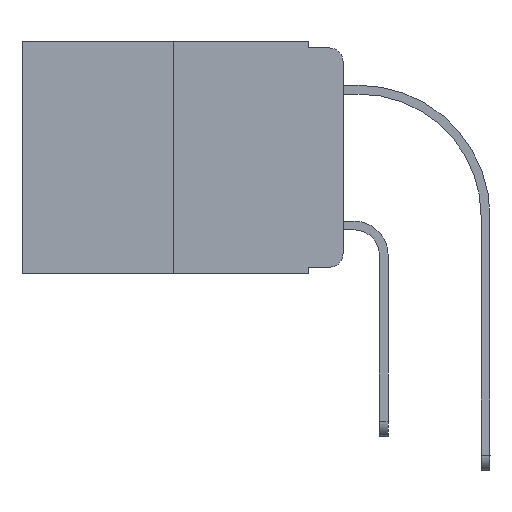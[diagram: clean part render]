
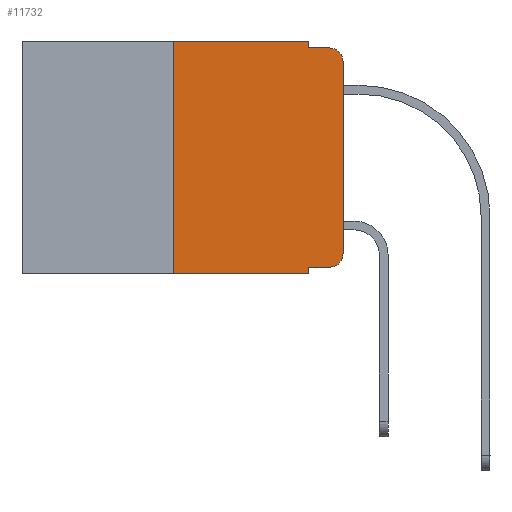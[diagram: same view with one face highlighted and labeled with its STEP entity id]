
A CAD part, left-side view. The second image highlights one B-rep face of the part: STEP entity #11732.
In plain terms, the highlighted planar face has unit normal (-1, 0, 0).
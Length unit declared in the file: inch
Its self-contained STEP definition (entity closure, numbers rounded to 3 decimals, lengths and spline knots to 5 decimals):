
#856 = ORIENTED_EDGE ( 'NONE', *, *, #9718, .F. ) ;
#1304 = EDGE_CURVE ( 'NONE', #6301, #11954, #2735, .T. ) ;
#1431 = EDGE_CURVE ( 'NONE', #22764, #14516, #23906, .T. ) ;
#1926 = DIRECTION ( 'NONE',  ( 0., 0., 1. ) ) ;
#2358 = AXIS2_PLACEMENT_3D ( 'NONE', #17321, #22872, #11988 ) ;
#2363 = DIRECTION ( 'NONE',  ( 0., 0., -1. ) ) ;
#2381 = CARTESIAN_POINT ( 'NONE',  ( 0., 0.02, -0.01 ) ) ;
#2456 = DIRECTION ( 'NONE',  ( -1., 0., 0. ) ) ;
#2527 = AXIS2_PLACEMENT_3D ( 'NONE', #20752, #18953, #2363 ) ;
#2655 = ORIENTED_EDGE ( 'NONE', *, *, #7202, .T. ) ;
#2735 = LINE ( 'NONE', #8079, #3494 ) ;
#2986 = LINE ( 'NONE', #15823, #6838 ) ;
#3075 = LINE ( 'NONE', #19781, #23325 ) ;
#3313 = DIRECTION ( 'NONE',  ( 0., -1., 0. ) ) ;
#3494 = VECTOR ( 'NONE', #6258, 39.37008 ) ;
#3755 = CARTESIAN_POINT ( 'NONE',  ( 0., 0.051, -0.333 ) ) ;
#4298 = FACE_OUTER_BOUND ( 'NONE', #11430, .T. ) ;
#4517 = EDGE_CURVE ( 'NONE', #23279, #20441, #9704, .T. ) ;
#4777 = DIRECTION ( 'NONE',  ( 0., 0., -1. ) ) ;
#4959 = CARTESIAN_POINT ( 'NONE',  ( 0., 0., -0.03 ) ) ;
#5026 = CARTESIAN_POINT ( 'NONE',  ( 0., 0.25, 0. ) ) ;
#5058 = DIRECTION ( 'NONE',  ( 0., 0., 1. ) ) ;
#5303 = VERTEX_POINT ( 'NONE', #19049 ) ;
#5310 = VECTOR ( 'NONE', #1926, 39.37008 ) ;
#6258 = DIRECTION ( 'NONE',  ( 0., -1., 0. ) ) ;
#6301 = VERTEX_POINT ( 'NONE', #22852 ) ;
#6594 = DIRECTION ( 'NONE',  ( 0., -1., 0. ) ) ;
#6620 = VERTEX_POINT ( 'NONE', #2381 ) ;
#6838 = VECTOR ( 'NONE', #5058, 39.37008 ) ;
#7202 = EDGE_CURVE ( 'NONE', #20441, #20588, #14857, .T. ) ;
#7598 = CARTESIAN_POINT ( 'NONE',  ( 0., 0.051, -0.01 ) ) ;
#8079 = CARTESIAN_POINT ( 'NONE',  ( 0., 0.473, -0.343 ) ) ;
#8536 = DIRECTION ( 'NONE',  ( 0., 0., -1. ) ) ;
#8720 = CARTESIAN_POINT ( 'NONE',  ( 0., 0.02, -0.333 ) ) ;
#9040 = VERTEX_POINT ( 'NONE', #7598 ) ;
#9572 = EDGE_CURVE ( 'NONE', #20588, #6620, #11547, .T. ) ;
#9633 = PLANE ( 'NONE',  #2527 ) ;
#9704 = CIRCLE ( 'NONE', #2358, 0.02 ) ;
#9718 = EDGE_CURVE ( 'NONE', #9040, #6620, #17713, .T. ) ;
#9840 = DIRECTION ( 'NONE',  ( 0., 0., -1. ) ) ;
#10265 = EDGE_CURVE ( 'NONE', #5303, #23279, #23596, .T. ) ;
#10583 = CARTESIAN_POINT ( 'NONE',  ( 0., 0.473, 0. ) ) ;
#10814 = VECTOR ( 'NONE', #11002, 39.37008 ) ;
#10950 = VECTOR ( 'NONE', #3313, 39.37008 ) ;
#11002 = DIRECTION ( 'NONE',  ( 0., -1., 0. ) ) ;
#11430 = EDGE_LOOP ( 'NONE', ( #2655, #15937, #856, #16898, #21971, #12486, #11492, #12411, #14481, #18625 ) ) ;
#11492 = ORIENTED_EDGE ( 'NONE', *, *, #1304, .T. ) ;
#11547 = CIRCLE ( 'NONE', #18522, 0.02 ) ;
#11732 = ADVANCED_FACE ( 'NONE', ( #4298 ), #9633, .F. ) ;
#11854 = EDGE_CURVE ( 'NONE', #14516, #9040, #21117, .T. ) ;
#11954 = VERTEX_POINT ( 'NONE', #16266 ) ;
#11988 = DIRECTION ( 'NONE',  ( 0., 0., -1. ) ) ;
#12411 = ORIENTED_EDGE ( 'NONE', *, *, #16034, .F. ) ;
#12486 = ORIENTED_EDGE ( 'NONE', *, *, #12649, .F. ) ;
#12649 = EDGE_CURVE ( 'NONE', #6301, #22764, #2986, .T. ) ;
#12928 = CARTESIAN_POINT ( 'NONE',  ( 0., 0., -0.313 ) ) ;
#13267 = CARTESIAN_POINT ( 'NONE',  ( 0., 0., 0. ) ) ;
#14481 = ORIENTED_EDGE ( 'NONE', *, *, #10265, .T. ) ;
#14516 = VERTEX_POINT ( 'NONE', #21281 ) ;
#14857 = LINE ( 'NONE', #13267, #5310 ) ;
#15417 = CARTESIAN_POINT ( 'NONE',  ( 0., 0.02, -0.03 ) ) ;
#15823 = CARTESIAN_POINT ( 'NONE',  ( 0., 0.25, 0. ) ) ;
#15890 = CARTESIAN_POINT ( 'NONE',  ( 0., 0.051, -0.01 ) ) ;
#15937 = ORIENTED_EDGE ( 'NONE', *, *, #9572, .T. ) ;
#16034 = EDGE_CURVE ( 'NONE', #5303, #11954, #3075, .T. ) ;
#16266 = CARTESIAN_POINT ( 'NONE',  ( 0., 0.051, -0.343 ) ) ;
#16898 = ORIENTED_EDGE ( 'NONE', *, *, #11854, .F. ) ;
#17321 = CARTESIAN_POINT ( 'NONE',  ( 0., 0.02, -0.313 ) ) ;
#17596 = CARTESIAN_POINT ( 'NONE',  ( 0., 0.051, 0. ) ) ;
#17713 = LINE ( 'NONE', #15890, #17742 ) ;
#17742 = VECTOR ( 'NONE', #6594, 39.37008 ) ;
#18522 = AXIS2_PLACEMENT_3D ( 'NONE', #15417, #2456, #9840 ) ;
#18625 = ORIENTED_EDGE ( 'NONE', *, *, #4517, .T. ) ;
#18953 = DIRECTION ( 'NONE',  ( 1., 0., 0. ) ) ;
#19049 = CARTESIAN_POINT ( 'NONE',  ( 0., 0.051, -0.333 ) ) ;
#19541 = VECTOR ( 'NONE', #4777, 39.37008 ) ;
#19781 = CARTESIAN_POINT ( 'NONE',  ( 0., 0.051, 0. ) ) ;
#20441 = VERTEX_POINT ( 'NONE', #12928 ) ;
#20588 = VERTEX_POINT ( 'NONE', #4959 ) ;
#20752 = CARTESIAN_POINT ( 'NONE',  ( 0., 0.473, 0. ) ) ;
#21117 = LINE ( 'NONE', #17596, #19541 ) ;
#21281 = CARTESIAN_POINT ( 'NONE',  ( 0., 0.051, 0. ) ) ;
#21971 = ORIENTED_EDGE ( 'NONE', *, *, #1431, .F. ) ;
#22764 = VERTEX_POINT ( 'NONE', #5026 ) ;
#22852 = CARTESIAN_POINT ( 'NONE',  ( 0., 0.25, -0.343 ) ) ;
#22872 = DIRECTION ( 'NONE',  ( -1., 0., 0. ) ) ;
#23279 = VERTEX_POINT ( 'NONE', #8720 ) ;
#23325 = VECTOR ( 'NONE', #8536, 39.37008 ) ;
#23596 = LINE ( 'NONE', #3755, #10814 ) ;
#23906 = LINE ( 'NONE', #10583, #10950 ) ;
